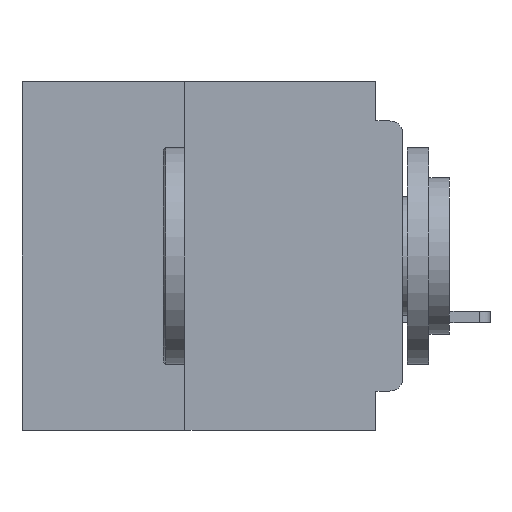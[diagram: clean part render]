
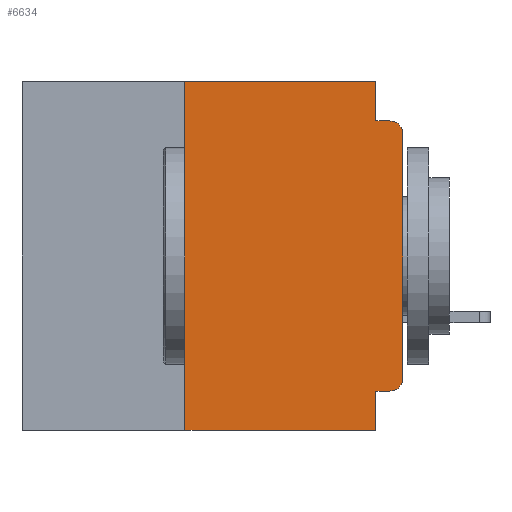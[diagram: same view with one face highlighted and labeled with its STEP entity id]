
A CAD part, left-side view. The second image highlights one B-rep face of the part: STEP entity #6634.
In plain terms, the highlighted planar face has unit normal (-1, 0, 0).
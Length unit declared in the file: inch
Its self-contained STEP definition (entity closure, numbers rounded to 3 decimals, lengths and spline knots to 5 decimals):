
#324 = CARTESIAN_POINT ( 'NONE',  ( 0., 0.437, -0.4 ) ) ;
#457 = VERTEX_POINT ( 'NONE', #53751 ) ;
#539 = DIRECTION ( 'NONE',  ( 0., -1., 0. ) ) ;
#633 = VERTEX_POINT ( 'NONE', #52344 ) ;
#658 = ORIENTED_EDGE ( 'NONE', *, *, #32631, .T. ) ;
#2640 = EDGE_CURVE ( 'NONE', #52494, #19298, #37614, .T. ) ;
#4880 = ORIENTED_EDGE ( 'NONE', *, *, #5069, .F. ) ;
#5069 = EDGE_CURVE ( 'NONE', #46787, #633, #25309, .T. ) ;
#5531 = EDGE_CURVE ( 'NONE', #13557, #457, #10387, .T. ) ;
#6634 = ADVANCED_FACE ( 'NONE', ( #7189 ), #17716, .F. ) ;
#7189 = FACE_OUTER_BOUND ( 'NONE', #22163, .T. ) ;
#7617 = ORIENTED_EDGE ( 'NONE', *, *, #64068, .T. ) ;
#8810 = VECTOR ( 'NONE', #8823, 39.37008 ) ;
#8823 = DIRECTION ( 'NONE',  ( 0., -1., 0. ) ) ;
#10198 = DIRECTION ( 'NONE',  ( 0., 0., 1. ) ) ;
#10387 = LINE ( 'NONE', #43508, #8810 ) ;
#10934 = AXIS2_PLACEMENT_3D ( 'NONE', #11245, #45847, #16321 ) ;
#11245 = CARTESIAN_POINT ( 'NONE',  ( 0., 0.015, -0.06 ) ) ;
#12239 = CARTESIAN_POINT ( 'NONE',  ( 0., 0.031, -0.355 ) ) ;
#13364 = LINE ( 'NONE', #46219, #28174 ) ;
#13517 = DIRECTION ( 'NONE',  ( 0., 0., -1. ) ) ;
#13557 = VERTEX_POINT ( 'NONE', #63672 ) ;
#14798 = CARTESIAN_POINT ( 'NONE',  ( 0., 0., -0.06 ) ) ;
#15475 = AXIS2_PLACEMENT_3D ( 'NONE', #50463, #20987, #55438 ) ;
#16321 = DIRECTION ( 'NONE',  ( 0., 0., -1. ) ) ;
#16705 = DIRECTION ( 'NONE',  ( 0., 0., -1. ) ) ;
#16766 = CARTESIAN_POINT ( 'NONE',  ( 0., 0., -0.355 ) ) ;
#17716 = PLANE ( 'NONE',  #36780 ) ;
#19298 = VERTEX_POINT ( 'NONE', #14798 ) ;
#20531 = EDGE_CURVE ( 'NONE', #46592, #52494, #46505, .T. ) ;
#20987 = DIRECTION ( 'NONE',  ( -1., 0., 0. ) ) ;
#22163 = EDGE_LOOP ( 'NONE', ( #43793, #658, #63840, #33375, #29769, #4880, #7617, #57577, #25040, #26056 ) ) ;
#23340 = CARTESIAN_POINT ( 'NONE',  ( 0., 0.031, -0.4 ) ) ;
#24403 = VECTOR ( 'NONE', #539, 39.37008 ) ;
#25040 = ORIENTED_EDGE ( 'NONE', *, *, #29436, .F. ) ;
#25309 = LINE ( 'NONE', #54748, #62993 ) ;
#26056 = ORIENTED_EDGE ( 'NONE', *, *, #20531, .T. ) ;
#26079 = EDGE_CURVE ( 'NONE', #633, #45816, #50549, .T. ) ;
#27688 = CARTESIAN_POINT ( 'NONE',  ( 0., 0.437, 0. ) ) ;
#28174 = VECTOR ( 'NONE', #16705, 39.37008 ) ;
#28279 = CARTESIAN_POINT ( 'NONE',  ( 0., 0.25, -0.4 ) ) ;
#29436 = EDGE_CURVE ( 'NONE', #46592, #63134, #58474, .T. ) ;
#29769 = ORIENTED_EDGE ( 'NONE', *, *, #26079, .F. ) ;
#30548 = CARTESIAN_POINT ( 'NONE',  ( 0., 0.031, 0. ) ) ;
#31970 = CARTESIAN_POINT ( 'NONE',  ( 0., 0.015, -0.355 ) ) ;
#32631 = EDGE_CURVE ( 'NONE', #19298, #457, #54322, .T. ) ;
#32670 = DIRECTION ( 'NONE',  ( 0., 0., -1. ) ) ;
#33375 = ORIENTED_EDGE ( 'NONE', *, *, #58797, .F. ) ;
#33921 = VECTOR ( 'NONE', #51236, 39.37008 ) ;
#34796 = CARTESIAN_POINT ( 'NONE',  ( 0., 0., -0.34 ) ) ;
#36091 = DIRECTION ( 'NONE',  ( 0., -1., 0. ) ) ;
#36780 = AXIS2_PLACEMENT_3D ( 'NONE', #27688, #62061, #32670 ) ;
#37510 = LINE ( 'NONE', #324, #24403 ) ;
#37614 = LINE ( 'NONE', #56593, #52184 ) ;
#38311 = CARTESIAN_POINT ( 'NONE',  ( 0., 0.031, -0.4 ) ) ;
#39639 = VECTOR ( 'NONE', #13517, 39.37008 ) ;
#43072 = EDGE_CURVE ( 'NONE', #63134, #53870, #52670, .T. ) ;
#43508 = CARTESIAN_POINT ( 'NONE',  ( 0., 0., -0.045 ) ) ;
#43793 = ORIENTED_EDGE ( 'NONE', *, *, #2640, .T. ) ;
#45816 = VERTEX_POINT ( 'NONE', #30548 ) ;
#45847 = DIRECTION ( 'NONE',  ( -1., 0., 0. ) ) ;
#45925 = CARTESIAN_POINT ( 'NONE',  ( 0., 0.437, 0. ) ) ;
#46219 = CARTESIAN_POINT ( 'NONE',  ( 0., 0.031, 0. ) ) ;
#46505 = CIRCLE ( 'NONE', #15475, 0.015 ) ;
#46592 = VERTEX_POINT ( 'NONE', #31970 ) ;
#46787 = VERTEX_POINT ( 'NONE', #28279 ) ;
#50463 = CARTESIAN_POINT ( 'NONE',  ( 0., 0.015, -0.34 ) ) ;
#50549 = LINE ( 'NONE', #45925, #60534 ) ;
#51236 = DIRECTION ( 'NONE',  ( 0., 1., 0. ) ) ;
#52184 = VECTOR ( 'NONE', #56803, 39.37008 ) ;
#52344 = CARTESIAN_POINT ( 'NONE',  ( 0., 0.25, 0. ) ) ;
#52494 = VERTEX_POINT ( 'NONE', #34796 ) ;
#52670 = LINE ( 'NONE', #23340, #39639 ) ;
#53751 = CARTESIAN_POINT ( 'NONE',  ( 0., 0.015, -0.045 ) ) ;
#53870 = VERTEX_POINT ( 'NONE', #38311 ) ;
#54322 = CIRCLE ( 'NONE', #10934, 0.015 ) ;
#54748 = CARTESIAN_POINT ( 'NONE',  ( 0., 0.25, -0.4 ) ) ;
#55438 = DIRECTION ( 'NONE',  ( 0., 0., -1. ) ) ;
#56593 = CARTESIAN_POINT ( 'NONE',  ( 0., 0., 0. ) ) ;
#56803 = DIRECTION ( 'NONE',  ( 0., 0., 1. ) ) ;
#57577 = ORIENTED_EDGE ( 'NONE', *, *, #43072, .F. ) ;
#58474 = LINE ( 'NONE', #16766, #33921 ) ;
#58797 = EDGE_CURVE ( 'NONE', #45816, #13557, #13364, .T. ) ;
#60534 = VECTOR ( 'NONE', #36091, 39.37008 ) ;
#62061 = DIRECTION ( 'NONE',  ( 1., 0., 0. ) ) ;
#62993 = VECTOR ( 'NONE', #10198, 39.37008 ) ;
#63134 = VERTEX_POINT ( 'NONE', #12239 ) ;
#63672 = CARTESIAN_POINT ( 'NONE',  ( 0., 0.031, -0.045 ) ) ;
#63840 = ORIENTED_EDGE ( 'NONE', *, *, #5531, .F. ) ;
#64068 = EDGE_CURVE ( 'NONE', #46787, #53870, #37510, .T. ) ;
